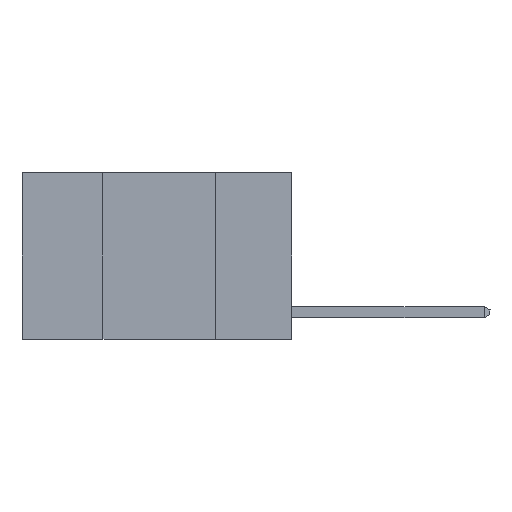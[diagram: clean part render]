
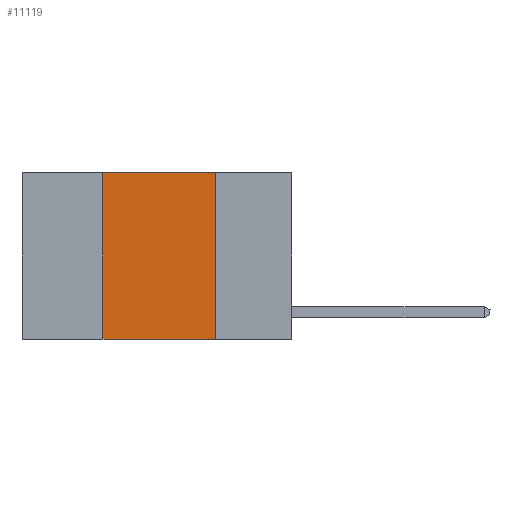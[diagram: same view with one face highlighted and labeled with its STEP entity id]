
A CAD part, left-side view. The second image highlights one B-rep face of the part: STEP entity #11119.
In plain terms, the highlighted planar face has unit normal (-1, 0, 0).
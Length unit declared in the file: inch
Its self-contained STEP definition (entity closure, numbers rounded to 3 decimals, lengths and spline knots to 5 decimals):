
#831 = DIRECTION ( 'NONE',  ( 1., 0., 0. ) ) ;
#959 = AXIS2_PLACEMENT_3D ( 'NONE', #14331, #831, #16545 ) ;
#960 = VERTEX_POINT ( 'NONE', #25231 ) ;
#1101 = VECTOR ( 'NONE', #12898, 39.37008 ) ;
#1200 = ORIENTED_EDGE ( 'NONE', *, *, #2738, .F. ) ;
#1806 = LINE ( 'NONE', #6122, #1101 ) ;
#2022 = VECTOR ( 'NONE', #24329, 39.37008 ) ;
#2738 = EDGE_CURVE ( 'NONE', #5334, #8162, #23877, .T. ) ;
#3610 = EDGE_CURVE ( 'NONE', #8162, #960, #21844, .T. ) ;
#4257 = ORIENTED_EDGE ( 'NONE', *, *, #21271, .F. ) ;
#5102 = VERTEX_POINT ( 'NONE', #5636 ) ;
#5334 = VERTEX_POINT ( 'NONE', #21971 ) ;
#5636 = CARTESIAN_POINT ( 'NONE',  ( 0., 0.17, -0.37 ) ) ;
#6122 = CARTESIAN_POINT ( 'NONE',  ( 0., 0.6, -0.37 ) ) ;
#6595 = CARTESIAN_POINT ( 'NONE',  ( 0., 0.17, 0. ) ) ;
#6790 = DIRECTION ( 'NONE',  ( 0., -1., 0. ) ) ;
#8162 = VERTEX_POINT ( 'NONE', #26605 ) ;
#9376 = VECTOR ( 'NONE', #6790, 39.37008 ) ;
#10623 = CARTESIAN_POINT ( 'NONE',  ( 0., 0.42, 0. ) ) ;
#11119 = ADVANCED_FACE ( 'NONE', ( #13162 ), #25227, .F. ) ;
#11332 = CARTESIAN_POINT ( 'NONE',  ( 0., 0.6, 0. ) ) ;
#11629 = EDGE_LOOP ( 'NONE', ( #4257, #26712, #1200, #20120 ) ) ;
#12898 = DIRECTION ( 'NONE',  ( 0., -1., 0. ) ) ;
#13162 = FACE_OUTER_BOUND ( 'NONE', #11629, .T. ) ;
#14331 = CARTESIAN_POINT ( 'NONE',  ( 0., 0.6, 0. ) ) ;
#16545 = DIRECTION ( 'NONE',  ( 0., 0., -1. ) ) ;
#18000 = VECTOR ( 'NONE', #23917, 39.37008 ) ;
#19912 = LINE ( 'NONE', #6595, #2022 ) ;
#20120 = ORIENTED_EDGE ( 'NONE', *, *, #25470, .T. ) ;
#21271 = EDGE_CURVE ( 'NONE', #960, #5102, #19912, .T. ) ;
#21844 = LINE ( 'NONE', #11332, #9376 ) ;
#21971 = CARTESIAN_POINT ( 'NONE',  ( 0., 0.42, -0.37 ) ) ;
#23877 = LINE ( 'NONE', #10623, #18000 ) ;
#23917 = DIRECTION ( 'NONE',  ( 0., 0., 1. ) ) ;
#24329 = DIRECTION ( 'NONE',  ( 0., 0., -1. ) ) ;
#25227 = PLANE ( 'NONE',  #959 ) ;
#25231 = CARTESIAN_POINT ( 'NONE',  ( 0., 0.17, 0. ) ) ;
#25470 = EDGE_CURVE ( 'NONE', #5334, #5102, #1806, .T. ) ;
#26605 = CARTESIAN_POINT ( 'NONE',  ( 0., 0.42, 0. ) ) ;
#26712 = ORIENTED_EDGE ( 'NONE', *, *, #3610, .F. ) ;
